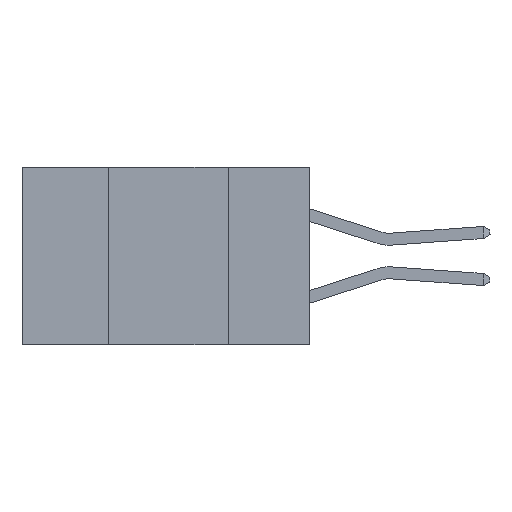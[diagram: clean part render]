
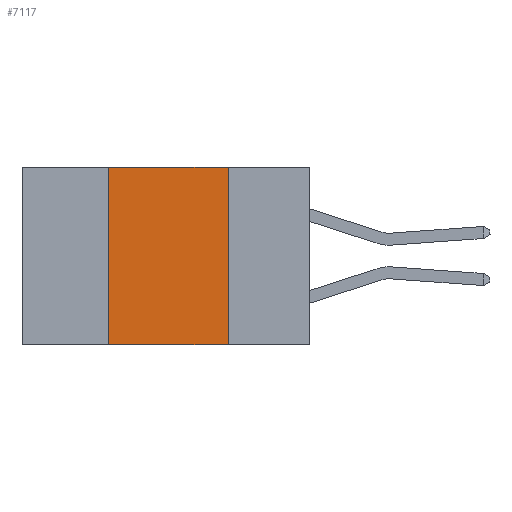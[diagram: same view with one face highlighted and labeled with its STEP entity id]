
A CAD part, left-side view. The second image highlights one B-rep face of the part: STEP entity #7117.
In plain terms, the highlighted planar face has unit normal (-1, 0, 0).
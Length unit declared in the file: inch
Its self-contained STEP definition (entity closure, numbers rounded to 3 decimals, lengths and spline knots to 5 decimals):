
#436 = EDGE_LOOP ( 'NONE', ( #19532, #27113, #24787, #3848 ) ) ;
#1534 = EDGE_CURVE ( 'NONE', #8659, #9909, #20107, .T. ) ;
#1687 = DIRECTION ( 'NONE',  ( 0., 0., -1. ) ) ;
#2315 = CARTESIAN_POINT ( 'NONE',  ( 0., 0.17, 0. ) ) ;
#2319 = LINE ( 'NONE', #24206, #24620 ) ;
#3503 = CARTESIAN_POINT ( 'NONE',  ( 0., 0.6, 0. ) ) ;
#3848 = ORIENTED_EDGE ( 'NONE', *, *, #18085, .T. ) ;
#4079 = CARTESIAN_POINT ( 'NONE',  ( 0., 0.17, 0. ) ) ;
#4484 = FACE_OUTER_BOUND ( 'NONE', #436, .T. ) ;
#4761 = VECTOR ( 'NONE', #1687, 39.37008 ) ;
#5188 = DIRECTION ( 'NONE',  ( 1., 0., 0. ) ) ;
#7117 = ADVANCED_FACE ( 'NONE', ( #4484 ), #18296, .F. ) ;
#7163 = LINE ( 'NONE', #11128, #14183 ) ;
#8659 = VERTEX_POINT ( 'NONE', #2315 ) ;
#8940 = VERTEX_POINT ( 'NONE', #21658 ) ;
#9909 = VERTEX_POINT ( 'NONE', #20549 ) ;
#11128 = CARTESIAN_POINT ( 'NONE',  ( 0., 0.6, -0.37 ) ) ;
#12964 = VERTEX_POINT ( 'NONE', #22112 ) ;
#14122 = CARTESIAN_POINT ( 'NONE',  ( 0., 0.6, 0. ) ) ;
#14183 = VECTOR ( 'NONE', #26163, 39.37008 ) ;
#15528 = DIRECTION ( 'NONE',  ( 0., 0., 1. ) ) ;
#16772 = VECTOR ( 'NONE', #22462, 39.37008 ) ;
#18085 = EDGE_CURVE ( 'NONE', #8940, #9909, #7163, .T. ) ;
#18296 = PLANE ( 'NONE',  #20070 ) ;
#19284 = EDGE_CURVE ( 'NONE', #12964, #8659, #23714, .T. ) ;
#19532 = ORIENTED_EDGE ( 'NONE', *, *, #1534, .F. ) ;
#20070 = AXIS2_PLACEMENT_3D ( 'NONE', #3503, #5188, #22231 ) ;
#20107 = LINE ( 'NONE', #4079, #4761 ) ;
#20549 = CARTESIAN_POINT ( 'NONE',  ( 0., 0.17, -0.37 ) ) ;
#21658 = CARTESIAN_POINT ( 'NONE',  ( 0., 0.42, -0.37 ) ) ;
#22112 = CARTESIAN_POINT ( 'NONE',  ( 0., 0.42, 0. ) ) ;
#22231 = DIRECTION ( 'NONE',  ( 0., 0., -1. ) ) ;
#22462 = DIRECTION ( 'NONE',  ( 0., -1., 0. ) ) ;
#23714 = LINE ( 'NONE', #14122, #16772 ) ;
#24203 = EDGE_CURVE ( 'NONE', #8940, #12964, #2319, .T. ) ;
#24206 = CARTESIAN_POINT ( 'NONE',  ( 0., 0.42, 0. ) ) ;
#24620 = VECTOR ( 'NONE', #15528, 39.37008 ) ;
#24787 = ORIENTED_EDGE ( 'NONE', *, *, #24203, .F. ) ;
#26163 = DIRECTION ( 'NONE',  ( 0., -1., 0. ) ) ;
#27113 = ORIENTED_EDGE ( 'NONE', *, *, #19284, .F. ) ;
